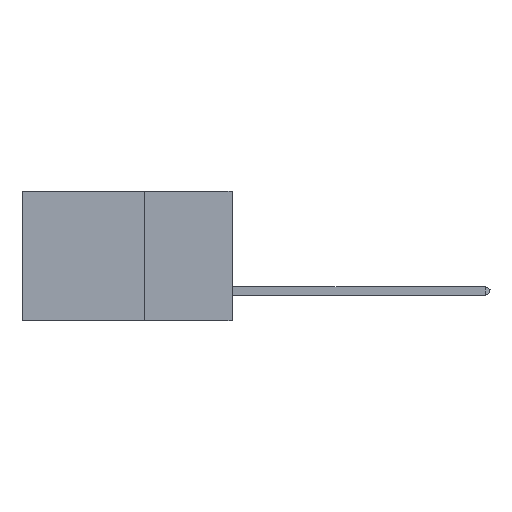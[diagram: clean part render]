
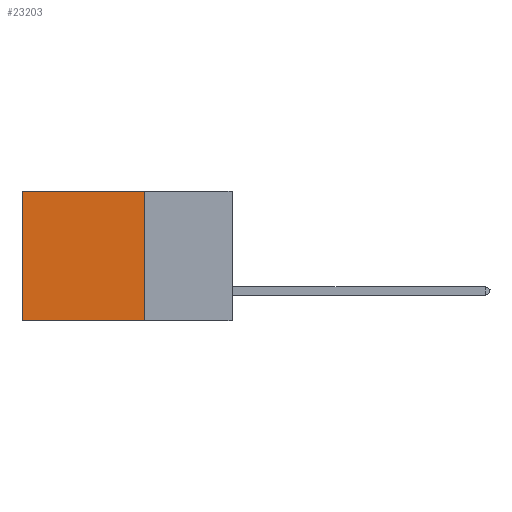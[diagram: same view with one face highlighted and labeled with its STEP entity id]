
A CAD part, left-side view. The second image highlights one B-rep face of the part: STEP entity #23203.
In plain terms, the highlighted planar face has unit normal (-1, 0, 0).
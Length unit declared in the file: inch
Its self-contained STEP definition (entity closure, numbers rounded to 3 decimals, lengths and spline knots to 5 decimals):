
#192 = CARTESIAN_POINT ( 'NONE',  ( 0.2875, 0.25, -0.37 ) ) ;
#502 = LINE ( 'NONE', #19511, #4838 ) ;
#708 = VECTOR ( 'NONE', #13335, 39.37008 ) ;
#861 = DIRECTION ( 'NONE',  ( 0., 1., 0. ) ) ;
#1188 = FACE_OUTER_BOUND ( 'NONE', #19984, .T. ) ;
#1994 = EDGE_CURVE ( 'NONE', #15866, #25402, #29463, .T. ) ;
#2343 = DIRECTION ( 'NONE',  ( 0., 1., 0. ) ) ;
#3748 = CARTESIAN_POINT ( 'NONE',  ( 0.2875, 0.25, 0. ) ) ;
#4117 = DIRECTION ( 'NONE',  ( 1., 0., 0. ) ) ;
#4838 = VECTOR ( 'NONE', #10332, 39.37008 ) ;
#5439 = LINE ( 'NONE', #16706, #22900 ) ;
#6522 = DIRECTION ( 'NONE',  ( 0., 0., -1. ) ) ;
#8865 = CARTESIAN_POINT ( 'NONE',  ( 0.2875, 0.25, 0. ) ) ;
#9529 = AXIS2_PLACEMENT_3D ( 'NONE', #8865, #4117, #6522 ) ;
#9779 = EDGE_CURVE ( 'NONE', #15866, #25689, #502, .T. ) ;
#10332 = DIRECTION ( 'NONE',  ( 0., 0., -1. ) ) ;
#11145 = ORIENTED_EDGE ( 'NONE', *, *, #1994, .T. ) ;
#11202 = PLANE ( 'NONE',  #9529 ) ;
#13335 = DIRECTION ( 'NONE',  ( 0., 0., -1. ) ) ;
#14366 = ORIENTED_EDGE ( 'NONE', *, *, #9779, .F. ) ;
#14633 = CARTESIAN_POINT ( 'NONE',  ( 0.2875, 0.6, 0. ) ) ;
#15521 = EDGE_CURVE ( 'NONE', #25689, #22883, #5439, .T. ) ;
#15866 = VERTEX_POINT ( 'NONE', #23559 ) ;
#15899 = VECTOR ( 'NONE', #2343, 39.37008 ) ;
#16068 = LINE ( 'NONE', #14633, #708 ) ;
#16706 = CARTESIAN_POINT ( 'NONE',  ( 0.2875, 0.25, -0.37 ) ) ;
#16779 = EDGE_CURVE ( 'NONE', #25402, #22883, #16068, .T. ) ;
#18275 = ORIENTED_EDGE ( 'NONE', *, *, #16779, .T. ) ;
#19511 = CARTESIAN_POINT ( 'NONE',  ( 0.2875, 0.25, 0. ) ) ;
#19578 = CARTESIAN_POINT ( 'NONE',  ( 0.2875, 0.6, 0. ) ) ;
#19984 = EDGE_LOOP ( 'NONE', ( #18275, #26662, #14366, #11145 ) ) ;
#22883 = VERTEX_POINT ( 'NONE', #26593 ) ;
#22900 = VECTOR ( 'NONE', #861, 39.37008 ) ;
#23203 = ADVANCED_FACE ( 'NONE', ( #1188 ), #11202, .F. ) ;
#23559 = CARTESIAN_POINT ( 'NONE',  ( 0.2875, 0.25, 0. ) ) ;
#25402 = VERTEX_POINT ( 'NONE', #19578 ) ;
#25689 = VERTEX_POINT ( 'NONE', #192 ) ;
#26593 = CARTESIAN_POINT ( 'NONE',  ( 0.2875, 0.6, -0.37 ) ) ;
#26662 = ORIENTED_EDGE ( 'NONE', *, *, #15521, .F. ) ;
#29463 = LINE ( 'NONE', #3748, #15899 ) ;
